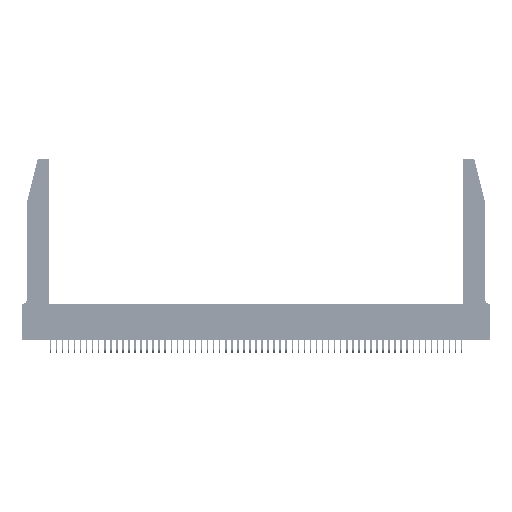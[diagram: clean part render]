
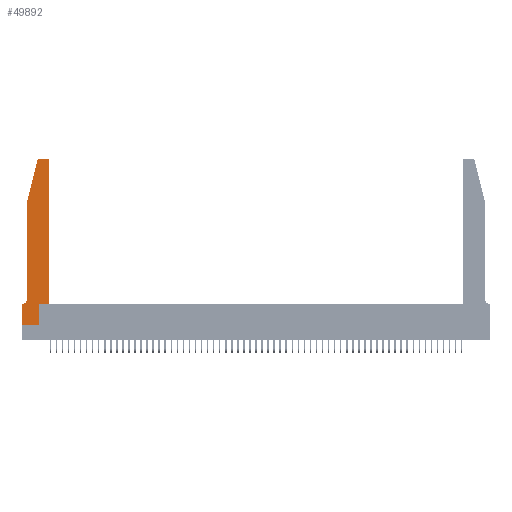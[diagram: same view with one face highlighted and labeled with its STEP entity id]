
A CAD part, top view. The second image highlights one B-rep face of the part: STEP entity #49892.
In plain terms, the highlighted planar face has unit normal (0, 0, 1).
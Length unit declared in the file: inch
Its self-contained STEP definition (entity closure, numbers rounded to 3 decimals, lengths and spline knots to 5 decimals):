
#452 = LINE ( 'NONE', #47709, #34182 ) ;
#534 = EDGE_CURVE ( 'NONE', #17870, #34084, #8136, .T. ) ;
#796 = DIRECTION ( 'NONE',  ( -1., 0., 0. ) ) ;
#1663 = CARTESIAN_POINT ( 'NONE',  ( 0.2605, 2.75, 0.37 ) ) ;
#1743 = VERTEX_POINT ( 'NONE', #10209 ) ;
#2288 = VERTEX_POINT ( 'NONE', #22502 ) ;
#3318 = EDGE_CURVE ( 'NONE', #5063, #10272, #6465, .T. ) ;
#3327 = CARTESIAN_POINT ( 'NONE',  ( 0.4505, 0.35, 0.37 ) ) ;
#3807 = DIRECTION ( 'NONE',  ( 1., 0., 0. ) ) ;
#5063 = VERTEX_POINT ( 'NONE', #26775 ) ;
#5359 = EDGE_CURVE ( 'NONE', #43477, #34991, #18654, .T. ) ;
#5430 = CARTESIAN_POINT ( 'NONE',  ( 0.0755, 2., 0.37 ) ) ;
#5603 = EDGE_CURVE ( 'NONE', #34991, #47678, #26815, .T. ) ;
#5756 = CIRCLE ( 'NONE', #36987, 0.07 ) ;
#6098 = DIRECTION ( 'NONE',  ( -1., 0., 0. ) ) ;
#6465 = CIRCLE ( 'NONE', #32723, 0.03 ) ;
#6942 = EDGE_CURVE ( 'NONE', #1743, #16367, #34432, .T. ) ;
#7337 = ORIENTED_EDGE ( 'NONE', *, *, #51169, .T. ) ;
#7747 = CARTESIAN_POINT ( 'NONE',  ( 0.284, 2.72, 0.37 ) ) ;
#7756 = CARTESIAN_POINT ( 'NONE',  ( 0.4505, 0.35, 0.37 ) ) ;
#7887 = CARTESIAN_POINT ( 'NONE',  ( 0., 0., 0.37 ) ) ;
#8136 = LINE ( 'NONE', #16812, #52121 ) ;
#8611 = VECTOR ( 'NONE', #6098, 39.37008 ) ;
#9047 = VERTEX_POINT ( 'NONE', #5430 ) ;
#9389 = DIRECTION ( 'NONE',  ( 0., 0., 1. ) ) ;
#10002 = LINE ( 'NONE', #1663, #8611 ) ;
#10209 = CARTESIAN_POINT ( 'NONE',  ( 0.2865, 0., 0.37 ) ) ;
#10272 = VERTEX_POINT ( 'NONE', #32086 ) ;
#10312 = AXIS2_PLACEMENT_3D ( 'NONE', #56485, #30178, #3807 ) ;
#10859 = ORIENTED_EDGE ( 'NONE', *, *, #56632, .T. ) ;
#11047 = VECTOR ( 'NONE', #48263, 39.37008 ) ;
#11690 = EDGE_CURVE ( 'NONE', #10272, #9047, #43417, .T. ) ;
#11837 = EDGE_CURVE ( 'NONE', #34084, #2288, #17371, .T. ) ;
#12195 = DIRECTION ( 'NONE',  ( 1., 0., 0. ) ) ;
#13967 = ORIENTED_EDGE ( 'NONE', *, *, #48600, .T. ) ;
#15332 = VECTOR ( 'NONE', #56738, 39.37008 ) ;
#15406 = CARTESIAN_POINT ( 'NONE',  ( 0.4505, 2.72, 0.37 ) ) ;
#15679 = ORIENTED_EDGE ( 'NONE', *, *, #5359, .T. ) ;
#15873 = ORIENTED_EDGE ( 'NONE', *, *, #5603, .T. ) ;
#16367 = VERTEX_POINT ( 'NONE', #17024 ) ;
#16547 = CARTESIAN_POINT ( 'NONE',  ( 0.0755, 0.42, 0.37 ) ) ;
#16730 = AXIS2_PLACEMENT_3D ( 'NONE', #35533, #9389, #40106 ) ;
#16812 = CARTESIAN_POINT ( 'NONE',  ( 0.0755, 0.35, 0.37 ) ) ;
#17024 = CARTESIAN_POINT ( 'NONE',  ( 0.2865, 0.35, 0.37 ) ) ;
#17371 = LINE ( 'NONE', #7887, #37949 ) ;
#17870 = VERTEX_POINT ( 'NONE', #32037 ) ;
#18654 = LINE ( 'NONE', #50502, #37821 ) ;
#20638 = EDGE_CURVE ( 'NONE', #9047, #53107, #50313, .T. ) ;
#21185 = DIRECTION ( 'NONE',  ( 0., -1., 0. ) ) ;
#21245 = ORIENTED_EDGE ( 'NONE', *, *, #3318, .T. ) ;
#22502 = CARTESIAN_POINT ( 'NONE',  ( 0., 0., 0.37 ) ) ;
#23339 = ORIENTED_EDGE ( 'NONE', *, *, #6942, .T. ) ;
#24766 = ORIENTED_EDGE ( 'NONE', *, *, #20638, .T. ) ;
#24863 = ORIENTED_EDGE ( 'NONE', *, *, #28616, .T. ) ;
#26775 = CARTESIAN_POINT ( 'NONE',  ( 0.284, 2.75, 0.37 ) ) ;
#26815 = CIRCLE ( 'NONE', #10312, 0.03 ) ;
#27151 = DIRECTION ( 'NONE',  ( 0., 0., -1. ) ) ;
#28616 = EDGE_CURVE ( 'NONE', #16367, #43477, #39350, .T. ) ;
#29222 = CARTESIAN_POINT ( 'NONE',  ( 0.4205, 2.75, 0.37 ) ) ;
#29266 = DIRECTION ( 'NONE',  ( -0.239, -0.971, 0. ) ) ;
#30178 = DIRECTION ( 'NONE',  ( 0., 0., 1. ) ) ;
#31801 = VECTOR ( 'NONE', #29266, 39.37008 ) ;
#32037 = CARTESIAN_POINT ( 'NONE',  ( 0.0055, 0.35, 0.37 ) ) ;
#32086 = CARTESIAN_POINT ( 'NONE',  ( 0.25487, 2.72718, 0.37 ) ) ;
#32723 = AXIS2_PLACEMENT_3D ( 'NONE', #7747, #38494, #12195 ) ;
#34084 = VERTEX_POINT ( 'NONE', #44443 ) ;
#34105 = DIRECTION ( 'NONE',  ( 1., 0., 0. ) ) ;
#34182 = VECTOR ( 'NONE', #34688, 39.37008 ) ;
#34432 = LINE ( 'NONE', #48074, #11047 ) ;
#34688 = DIRECTION ( 'NONE',  ( 1., 0., 0. ) ) ;
#34991 = VERTEX_POINT ( 'NONE', #15406 ) ;
#35533 = CARTESIAN_POINT ( 'NONE',  ( 0., 0.35, 0.37 ) ) ;
#35759 = ORIENTED_EDGE ( 'NONE', *, *, #11837, .T. ) ;
#36987 = AXIS2_PLACEMENT_3D ( 'NONE', #53448, #27151, #796 ) ;
#37821 = VECTOR ( 'NONE', #54963, 39.37008 ) ;
#37949 = VECTOR ( 'NONE', #21185, 39.37008 ) ;
#38431 = ORIENTED_EDGE ( 'NONE', *, *, #534, .T. ) ;
#38494 = DIRECTION ( 'NONE',  ( 0., 0., 1. ) ) ;
#39350 = LINE ( 'NONE', #3327, #40745 ) ;
#40106 = DIRECTION ( 'NONE',  ( 1., 0., 0. ) ) ;
#40745 = VECTOR ( 'NONE', #34105, 39.37008 ) ;
#43417 = LINE ( 'NONE', #46698, #31801 ) ;
#43477 = VERTEX_POINT ( 'NONE', #7756 ) ;
#44443 = CARTESIAN_POINT ( 'NONE',  ( 0., 0.35, 0.37 ) ) ;
#46698 = CARTESIAN_POINT ( 'NONE',  ( 0.0755, 2., 0.37 ) ) ;
#47030 = FACE_OUTER_BOUND ( 'NONE', #53681, .T. ) ;
#47678 = VERTEX_POINT ( 'NONE', #29222 ) ;
#47709 = CARTESIAN_POINT ( 'NONE',  ( 0., 0., 0.37 ) ) ;
#48023 = ORIENTED_EDGE ( 'NONE', *, *, #11690, .T. ) ;
#48074 = CARTESIAN_POINT ( 'NONE',  ( 0.2865, 0.35, 0.37 ) ) ;
#48263 = DIRECTION ( 'NONE',  ( 0., 1., 0. ) ) ;
#48600 = EDGE_CURVE ( 'NONE', #2288, #1743, #452, .T. ) ;
#49892 = ADVANCED_FACE ( 'NONE', ( #47030 ), #53181, .T. ) ;
#50313 = LINE ( 'NONE', #52297, #15332 ) ;
#50502 = CARTESIAN_POINT ( 'NONE',  ( 0.4505, 0.35, 0.37 ) ) ;
#51169 = EDGE_CURVE ( 'NONE', #53107, #17870, #5756, .T. ) ;
#52121 = VECTOR ( 'NONE', #56339, 39.37008 ) ;
#52297 = CARTESIAN_POINT ( 'NONE',  ( 0.0755, 2., 0.37 ) ) ;
#53107 = VERTEX_POINT ( 'NONE', #16547 ) ;
#53181 = PLANE ( 'NONE',  #16730 ) ;
#53448 = CARTESIAN_POINT ( 'NONE',  ( 0.0055, 0.42, 0.37 ) ) ;
#53681 = EDGE_LOOP ( 'NONE', ( #10859, #21245, #48023, #24766, #7337, #38431, #35759, #13967, #23339, #24863, #15679, #15873 ) ) ;
#54963 = DIRECTION ( 'NONE',  ( 0., 1., 0. ) ) ;
#56339 = DIRECTION ( 'NONE',  ( -1., 0., 0. ) ) ;
#56485 = CARTESIAN_POINT ( 'NONE',  ( 0.4205, 2.72, 0.37 ) ) ;
#56632 = EDGE_CURVE ( 'NONE', #47678, #5063, #10002, .T. ) ;
#56738 = DIRECTION ( 'NONE',  ( 0., -1., 0. ) ) ;
